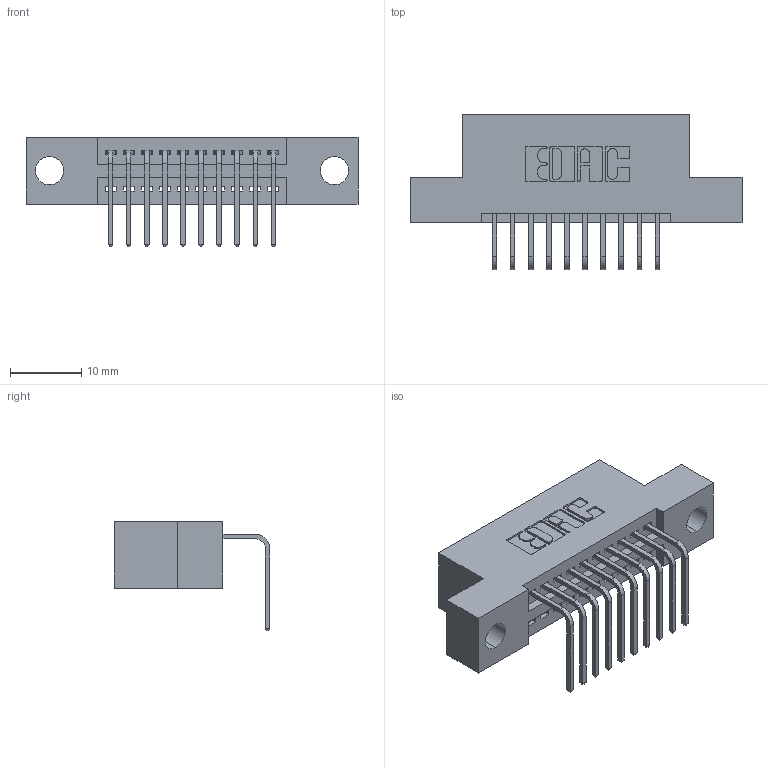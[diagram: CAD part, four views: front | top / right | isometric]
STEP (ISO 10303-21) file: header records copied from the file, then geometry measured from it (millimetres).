
FILE_DESCRIPTION (( 'STEP AP203' ), '1' );
FILE_NAME ('345-010-558-104.STEP', '2021-06-01T16:11:39', ( '' ), ( '' ), 'SwSTEP 2.0', 'SolidWorks 2020', '' );
FILE_SCHEMA (( 'CONFIG_CONTROL_DESIGN' ));
Length unit declared in the file: inch
Products named in the file (3): 345-010-558-104; 345 Part_Flush Mounting Lugs - 0.156 Dia-TI; 345-292-001_558 Tail - 2
Assembly tree (11 placements, depth 2):
  345-010-558-104
    345 Part_Flush Mounting Lugs - 0.156 Dia-TI
    345-292-001_558 Tail - 2  x10
Bounding box: 46.61 x 21.83 x 15.37 mm (x, y, z)
Volume: 4092.2 mm3; surface area: 5041.5 mm2
Topology: 11 solids, 11 shells, 740 faces, 2197 edges, 1450 vertices
Faces by surface type: plane 514, cylinder 226
Entity records: 12337 total; most frequent: CARTESIAN_POINT 2148, ORIENTED_EDGE 2090, DIRECTION 1921, EDGE_CURVE 1045, VECTOR 873, LINE 873, VERTEX_POINT 694, AXIS2_PLACEMENT_3D 524
